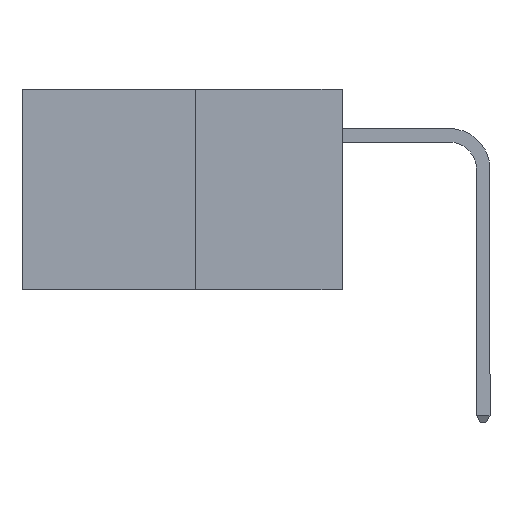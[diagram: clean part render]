
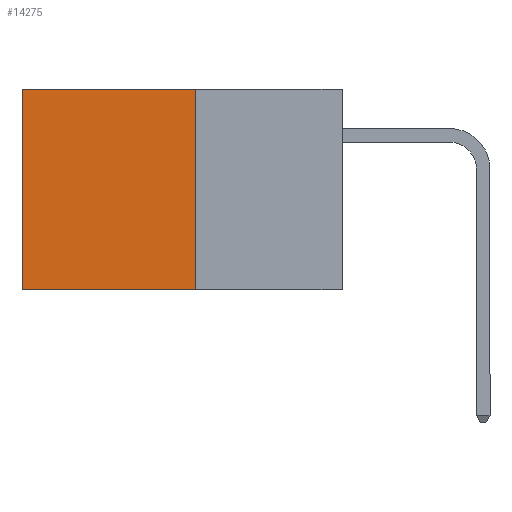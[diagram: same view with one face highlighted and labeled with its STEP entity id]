
A CAD part, left-side view. The second image highlights one B-rep face of the part: STEP entity #14275.
In plain terms, the highlighted planar face has unit normal (-1, 0, 0).
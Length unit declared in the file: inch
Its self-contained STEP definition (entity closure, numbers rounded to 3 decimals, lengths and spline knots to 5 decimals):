
#231 = CARTESIAN_POINT ( 'NONE',  ( 0.277, 0.27, -0.37 ) ) ;
#428 = LINE ( 'NONE', #11988, #21243 ) ;
#2838 = CARTESIAN_POINT ( 'NONE',  ( 0.277, 0.27, 0. ) ) ;
#3174 = VERTEX_POINT ( 'NONE', #12988 ) ;
#3214 = VERTEX_POINT ( 'NONE', #11267 ) ;
#3794 = EDGE_CURVE ( 'NONE', #4478, #3174, #5996, .T. ) ;
#4022 = LINE ( 'NONE', #10685, #16707 ) ;
#4315 = ORIENTED_EDGE ( 'NONE', *, *, #3794, .F. ) ;
#4478 = VERTEX_POINT ( 'NONE', #231 ) ;
#5858 = VERTEX_POINT ( 'NONE', #12543 ) ;
#5923 = EDGE_CURVE ( 'NONE', #3214, #4478, #4022, .T. ) ;
#5996 = LINE ( 'NONE', #9142, #14803 ) ;
#6766 = CARTESIAN_POINT ( 'NONE',  ( 0.277, 0.27, -0.37 ) ) ;
#6784 = ORIENTED_EDGE ( 'NONE', *, *, #13830, .T. ) ;
#8473 = DIRECTION ( 'NONE',  ( 0., 0., -1. ) ) ;
#9142 = CARTESIAN_POINT ( 'NONE',  ( 0.277, 0.27, -0.37 ) ) ;
#10664 = DIRECTION ( 'NONE',  ( 0., 0., -1. ) ) ;
#10685 = CARTESIAN_POINT ( 'NONE',  ( 0.277, 0.27, -0.37 ) ) ;
#11267 = CARTESIAN_POINT ( 'NONE',  ( 0.277, 0.27, 0. ) ) ;
#11988 = CARTESIAN_POINT ( 'NONE',  ( 0.277, 0.59, -0.37 ) ) ;
#12339 = DIRECTION ( 'NONE',  ( 0., 1., 0. ) ) ;
#12543 = CARTESIAN_POINT ( 'NONE',  ( 0.277, 0.59, 0. ) ) ;
#12662 = AXIS2_PLACEMENT_3D ( 'NONE', #6766, #18182, #8473 ) ;
#12979 = LINE ( 'NONE', #2838, #20499 ) ;
#12988 = CARTESIAN_POINT ( 'NONE',  ( 0.277, 0.59, -0.37 ) ) ;
#13830 = EDGE_CURVE ( 'NONE', #5858, #3174, #428, .T. ) ;
#14096 = EDGE_CURVE ( 'NONE', #3214, #5858, #12979, .T. ) ;
#14275 = ADVANCED_FACE ( 'NONE', ( #17497 ), #14997, .F. ) ;
#14803 = VECTOR ( 'NONE', #12339, 39.37008 ) ;
#14997 = PLANE ( 'NONE',  #12662 ) ;
#16707 = VECTOR ( 'NONE', #10664, 39.37008 ) ;
#16902 = DIRECTION ( 'NONE',  ( 0., 0., -1. ) ) ;
#17459 = ORIENTED_EDGE ( 'NONE', *, *, #5923, .F. ) ;
#17497 = FACE_OUTER_BOUND ( 'NONE', #19904, .T. ) ;
#17777 = DIRECTION ( 'NONE',  ( 0., 1., 0. ) ) ;
#18182 = DIRECTION ( 'NONE',  ( 1., 0., 0. ) ) ;
#19904 = EDGE_LOOP ( 'NONE', ( #6784, #4315, #17459, #20144 ) ) ;
#20144 = ORIENTED_EDGE ( 'NONE', *, *, #14096, .T. ) ;
#20499 = VECTOR ( 'NONE', #17777, 39.37008 ) ;
#21243 = VECTOR ( 'NONE', #16902, 39.37008 ) ;
